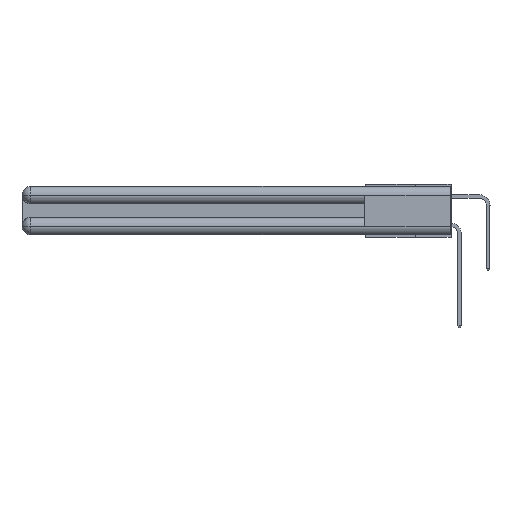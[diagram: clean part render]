
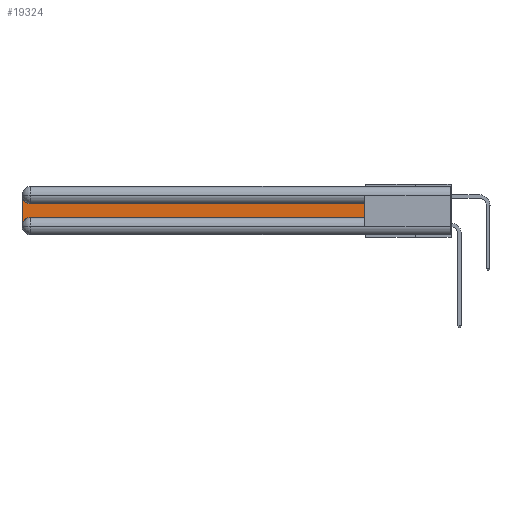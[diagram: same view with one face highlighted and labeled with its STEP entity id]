
A CAD part, left-side view. The second image highlights one B-rep face of the part: STEP entity #19324.
In plain terms, the highlighted planar face has unit normal (-1, 0, 0).
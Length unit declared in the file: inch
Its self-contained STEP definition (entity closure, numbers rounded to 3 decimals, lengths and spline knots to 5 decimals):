
#980 = CARTESIAN_POINT ( 'NONE',  ( 0.075, 3., -0.1225 ) ) ;
#1564 = EDGE_LOOP ( 'NONE', ( #27434, #28454, #20260, #18338, #24155, #32021 ) ) ;
#2198 = AXIS2_PLACEMENT_3D ( 'NONE', #19095, #32922, #5524 ) ;
#2574 = VERTEX_POINT ( 'NONE', #24879 ) ;
#3627 = CARTESIAN_POINT ( 'NONE',  ( 0.075, 2.94, -0.2175 ) ) ;
#4865 = LINE ( 'NONE', #34890, #33360 ) ;
#5524 = DIRECTION ( 'NONE',  ( 0., 0., -1. ) ) ;
#6091 = EDGE_CURVE ( 'NONE', #18994, #34463, #9895, .T. ) ;
#6161 = CARTESIAN_POINT ( 'NONE',  ( 0.075, 0.6, -0.2175 ) ) ;
#6171 = CARTESIAN_POINT ( 'NONE',  ( 0.075, 3., -0.2175 ) ) ;
#6209 = VECTOR ( 'NONE', #20137, 39.37008 ) ;
#9895 = LINE ( 'NONE', #6171, #14148 ) ;
#10209 = DIRECTION ( 'NONE',  ( 0., 1., 0. ) ) ;
#11818 = CARTESIAN_POINT ( 'NONE',  ( 0.075, 0.6, -0.1225 ) ) ;
#11871 = CARTESIAN_POINT ( 'NONE',  ( 0.075, 0.6, -0.2175 ) ) ;
#12345 = CARTESIAN_POINT ( 'NONE',  ( 0.075, 3., -0.0625 ) ) ;
#12842 = EDGE_CURVE ( 'NONE', #16208, #16393, #35133, .T. ) ;
#13701 = DIRECTION ( 'NONE',  ( 0., -1., 0. ) ) ;
#14148 = VECTOR ( 'NONE', #20267, 39.37008 ) ;
#15231 = CIRCLE ( 'NONE', #26873, 0.06 ) ;
#16041 = CIRCLE ( 'NONE', #2198, 0.06 ) ;
#16208 = VERTEX_POINT ( 'NONE', #3627 ) ;
#16218 = CARTESIAN_POINT ( 'NONE',  ( 0.075, 0.6, -0.2175 ) ) ;
#16393 = VERTEX_POINT ( 'NONE', #11871 ) ;
#16423 = AXIS2_PLACEMENT_3D ( 'NONE', #980, #20111, #28600 ) ;
#17358 = FACE_OUTER_BOUND ( 'NONE', #1564, .T. ) ;
#18338 = ORIENTED_EDGE ( 'NONE', *, *, #19674, .T. ) ;
#18566 = EDGE_CURVE ( 'NONE', #16393, #31939, #32593, .T. ) ;
#18994 = VERTEX_POINT ( 'NONE', #12345 ) ;
#19095 = CARTESIAN_POINT ( 'NONE',  ( 0.075, 2.94, -0.2775 ) ) ;
#19219 = CARTESIAN_POINT ( 'NONE',  ( 0.075, 3., -0.2775 ) ) ;
#19324 = ADVANCED_FACE ( 'NONE', ( #17358 ), #25573, .F. ) ;
#19674 = EDGE_CURVE ( 'NONE', #34463, #16208, #16041, .T. ) ;
#20111 = DIRECTION ( 'NONE',  ( 1., 0., 0. ) ) ;
#20137 = DIRECTION ( 'NONE',  ( 0., 0., 1. ) ) ;
#20260 = ORIENTED_EDGE ( 'NONE', *, *, #6091, .T. ) ;
#20267 = DIRECTION ( 'NONE',  ( 0., 0., -1. ) ) ;
#21526 = DIRECTION ( 'NONE',  ( 0., 0., -1. ) ) ;
#21568 = EDGE_CURVE ( 'NONE', #31939, #2574, #4865, .T. ) ;
#24155 = ORIENTED_EDGE ( 'NONE', *, *, #12842, .T. ) ;
#24879 = CARTESIAN_POINT ( 'NONE',  ( 0.075, 2.94, -0.1225 ) ) ;
#25573 = PLANE ( 'NONE',  #16423 ) ;
#26873 = AXIS2_PLACEMENT_3D ( 'NONE', #32514, #35643, #21526 ) ;
#26905 = VECTOR ( 'NONE', #13701, 39.37008 ) ;
#27434 = ORIENTED_EDGE ( 'NONE', *, *, #21568, .T. ) ;
#28454 = ORIENTED_EDGE ( 'NONE', *, *, #28921, .T. ) ;
#28600 = DIRECTION ( 'NONE',  ( 0., 0., -1. ) ) ;
#28921 = EDGE_CURVE ( 'NONE', #2574, #18994, #15231, .T. ) ;
#31939 = VERTEX_POINT ( 'NONE', #11818 ) ;
#32021 = ORIENTED_EDGE ( 'NONE', *, *, #18566, .T. ) ;
#32514 = CARTESIAN_POINT ( 'NONE',  ( 0.075, 2.94, -0.0625 ) ) ;
#32593 = LINE ( 'NONE', #6161, #6209 ) ;
#32922 = DIRECTION ( 'NONE',  ( 1., 0., 0. ) ) ;
#33360 = VECTOR ( 'NONE', #10209, 39.37008 ) ;
#34463 = VERTEX_POINT ( 'NONE', #19219 ) ;
#34890 = CARTESIAN_POINT ( 'NONE',  ( 0.075, 0.6, -0.1225 ) ) ;
#35133 = LINE ( 'NONE', #16218, #26905 ) ;
#35643 = DIRECTION ( 'NONE',  ( 1., 0., 0. ) ) ;
